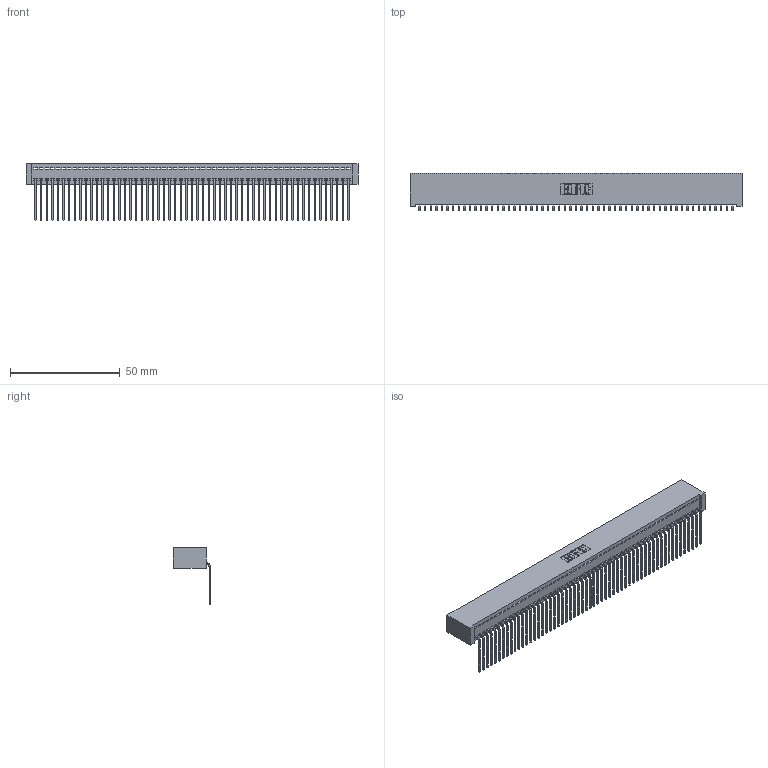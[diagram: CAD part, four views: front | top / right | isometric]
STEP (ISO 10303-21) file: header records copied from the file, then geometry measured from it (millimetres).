
FILE_DESCRIPTION (( 'STEP AP203' ), '1' );
FILE_NAME ('342-057-559-101.STEP', '2019-10-03T12:14:25', ( '' ), ( '' ), 'SwSTEP 2.0', 'SolidWorks 2016', '' );
FILE_SCHEMA (( 'CONFIG_CONTROL_DESIGN' ));
Length unit declared in the file: inch
Products named in the file (3): 342 Part_Lugless; 345-292-001_558 559 Tail - 1; 342-057-559-101
Assembly tree (58 placements, depth 2):
  342-057-559-101
    342 Part_Lugless
    345-292-001_558 559 Tail - 1  x57
Bounding box: 151.03 x 16.83 x 25.78 mm (x, y, z)
Volume: 13896.3 mm3; surface area: 22088 mm2
Topology: 58 solids, 58 shells, 3522 faces, 10649 edges, 7022 vertices
Faces by surface type: plane 2570, cylinder 952
Entity records: 32581 total; most frequent: CARTESIAN_POINT 5625, ORIENTED_EDGE 5618, DIRECTION 4707, EDGE_CURVE 2809, LINE 2689, VECTOR 2689, VERTEX_POINT 1870, AXIS2_PLACEMENT_3D 1009
